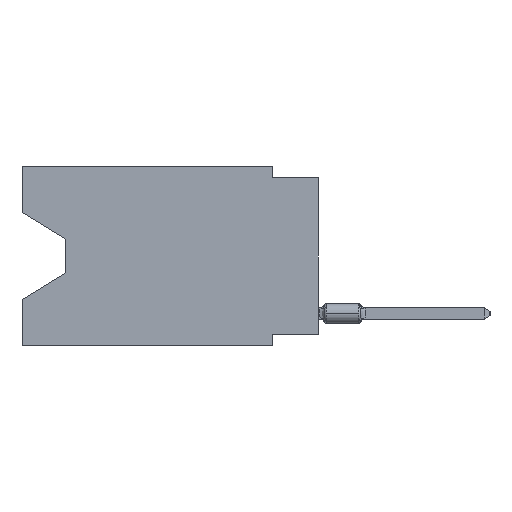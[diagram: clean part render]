
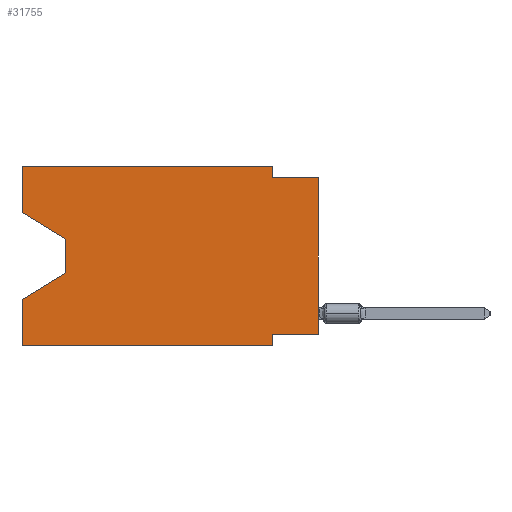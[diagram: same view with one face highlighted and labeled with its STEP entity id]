
A CAD part, left-side view. The second image highlights one B-rep face of the part: STEP entity #31755.
In plain terms, the highlighted planar face has unit normal (-1, 0, 0).
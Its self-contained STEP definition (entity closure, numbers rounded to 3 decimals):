
#3 = CARTESIAN_POINT ( 'NONE',  ( 0., 16.383, -2.546 ) ) ;
#266 = DIRECTION ( 'NONE',  ( 0., 0.855, -0.519 ) ) ;
#741 = EDGE_CURVE ( 'NONE', #55775, #19733, #58046, .T. ) ;
#993 = EDGE_CURVE ( 'NONE', #16217, #6384, #21470, .T. ) ;
#4747 = VECTOR ( 'NONE', #56675, 1000. ) ;
#5425 = EDGE_CURVE ( 'NONE', #16217, #34141, #39966, .T. ) ;
#5460 = EDGE_CURVE ( 'NONE', #55775, #35177, #15376, .T. ) ;
#5463 = CARTESIAN_POINT ( 'NONE',  ( 0., 2.54, 0. ) ) ;
#5688 = EDGE_CURVE ( 'NONE', #6384, #24599, #43544, .T. ) ;
#6215 = CARTESIAN_POINT ( 'NONE',  ( 0., 0., 0. ) ) ;
#6384 = VERTEX_POINT ( 'NONE', #26692 ) ;
#6504 = ORIENTED_EDGE ( 'NONE', *, *, #25379, .F. ) ;
#6637 = VERTEX_POINT ( 'NONE', #59790 ) ;
#7893 = DIRECTION ( 'NONE',  ( 0., 0., 1. ) ) ;
#8141 = LINE ( 'NONE', #43178, #21584 ) ;
#9099 = DIRECTION ( 'NONE',  ( 0., 0., -1. ) ) ;
#9825 = FACE_OUTER_BOUND ( 'NONE', #24979, .T. ) ;
#10461 = PLANE ( 'NONE',  #39262 ) ;
#12019 = CARTESIAN_POINT ( 'NONE',  ( 0., 16.383, -7.36 ) ) ;
#13508 = DIRECTION ( 'NONE',  ( 1., 0., 0. ) ) ;
#14356 = CARTESIAN_POINT ( 'NONE',  ( 0., 16.383, 0. ) ) ;
#14733 = VERTEX_POINT ( 'NONE', #24044 ) ;
#15062 = DIRECTION ( 'NONE',  ( 0., -0.855, -0.519 ) ) ;
#15376 = LINE ( 'NONE', #6215, #58860 ) ;
#15592 = LINE ( 'NONE', #5463, #54317 ) ;
#16217 = VERTEX_POINT ( 'NONE', #50211 ) ;
#17192 = CARTESIAN_POINT ( 'NONE',  ( 0., 16.383, 0. ) ) ;
#17951 = CARTESIAN_POINT ( 'NONE',  ( 0., 2.54, 0. ) ) ;
#18900 = DIRECTION ( 'NONE',  ( 0., -1., 0. ) ) ;
#19038 = VECTOR ( 'NONE', #53712, 1000. ) ;
#19636 = VERTEX_POINT ( 'NONE', #12019 ) ;
#19733 = VERTEX_POINT ( 'NONE', #49685 ) ;
#20646 = EDGE_CURVE ( 'NONE', #19733, #6637, #49858, .T. ) ;
#21047 = DIRECTION ( 'NONE',  ( 0., -1., 0. ) ) ;
#21470 = LINE ( 'NONE', #17192, #53207 ) ;
#21584 = VECTOR ( 'NONE', #18900, 1000. ) ;
#22934 = LINE ( 'NONE', #58698, #28875 ) ;
#23372 = ORIENTED_EDGE ( 'NONE', *, *, #61097, .T. ) ;
#23445 = ORIENTED_EDGE ( 'NONE', *, *, #51139, .T. ) ;
#23600 = EDGE_CURVE ( 'NONE', #24599, #28301, #15592, .T. ) ;
#23714 = ORIENTED_EDGE ( 'NONE', *, *, #49152, .F. ) ;
#24044 = CARTESIAN_POINT ( 'NONE',  ( 0., 13.97, -5.893 ) ) ;
#24599 = VERTEX_POINT ( 'NONE', #17951 ) ;
#24910 = CARTESIAN_POINT ( 'NONE',  ( 0., 2.54, -9.906 ) ) ;
#24979 = EDGE_LOOP ( 'NONE', ( #38047, #23445, #23372, #23714, #28029, #46603, #27506, #29976, #6504, #38285, #33761, #47927 ) ) ;
#25207 = CARTESIAN_POINT ( 'NONE',  ( 0., 0., -0.635 ) ) ;
#25379 = EDGE_CURVE ( 'NONE', #28301, #35177, #42009, .T. ) ;
#25544 = DIRECTION ( 'NONE',  ( 0., 0., 1. ) ) ;
#26692 = CARTESIAN_POINT ( 'NONE',  ( 0., 16.383, 0. ) ) ;
#27506 = ORIENTED_EDGE ( 'NONE', *, *, #741, .F. ) ;
#28029 = ORIENTED_EDGE ( 'NONE', *, *, #52487, .T. ) ;
#28301 = VERTEX_POINT ( 'NONE', #39928 ) ;
#28875 = VECTOR ( 'NONE', #7893, 1000. ) ;
#29799 = CARTESIAN_POINT ( 'NONE',  ( 0., 16.383, 0. ) ) ;
#29976 = ORIENTED_EDGE ( 'NONE', *, *, #5460, .T. ) ;
#31755 = ADVANCED_FACE ( 'NONE', ( #9825 ), #10461, .F. ) ;
#33484 = DIRECTION ( 'NONE',  ( 0., 0., -1. ) ) ;
#33761 = ORIENTED_EDGE ( 'NONE', *, *, #5688, .F. ) ;
#34141 = VERTEX_POINT ( 'NONE', #64300 ) ;
#34325 = VECTOR ( 'NONE', #43249, 1000. ) ;
#35177 = VERTEX_POINT ( 'NONE', #25207 ) ;
#35387 = CARTESIAN_POINT ( 'NONE',  ( 0., 0., -9.271 ) ) ;
#37346 = CARTESIAN_POINT ( 'NONE',  ( 0., 0., -9.271 ) ) ;
#38047 = ORIENTED_EDGE ( 'NONE', *, *, #5425, .T. ) ;
#38285 = ORIENTED_EDGE ( 'NONE', *, *, #23600, .F. ) ;
#39262 = AXIS2_PLACEMENT_3D ( 'NONE', #29799, #13508, #33484 ) ;
#39928 = CARTESIAN_POINT ( 'NONE',  ( 0., 2.54, -0.635 ) ) ;
#39966 = LINE ( 'NONE', #3, #53649 ) ;
#41779 = CARTESIAN_POINT ( 'NONE',  ( 0., 16.383, -9.906 ) ) ;
#41786 = DIRECTION ( 'NONE',  ( 0., 0., 1. ) ) ;
#42009 = LINE ( 'NONE', #61105, #47117 ) ;
#42565 = VECTOR ( 'NONE', #45898, 1000. ) ;
#43178 = CARTESIAN_POINT ( 'NONE',  ( 0., 16.383, -9.906 ) ) ;
#43249 = DIRECTION ( 'NONE',  ( 0., 1., 0. ) ) ;
#43544 = LINE ( 'NONE', #14356, #19038 ) ;
#44311 = VECTOR ( 'NONE', #266, 1000. ) ;
#45164 = CARTESIAN_POINT ( 'NONE',  ( 0., 13.97, -5.893 ) ) ;
#45898 = DIRECTION ( 'NONE',  ( 0., 0., -1. ) ) ;
#46603 = ORIENTED_EDGE ( 'NONE', *, *, #20646, .F. ) ;
#47117 = VECTOR ( 'NONE', #21047, 1000. ) ;
#47927 = ORIENTED_EDGE ( 'NONE', *, *, #993, .F. ) ;
#49147 = LINE ( 'NONE', #45164, #44311 ) ;
#49152 = EDGE_CURVE ( 'NONE', #58137, #19636, #22934, .T. ) ;
#49685 = CARTESIAN_POINT ( 'NONE',  ( 0., 2.54, -9.271 ) ) ;
#49858 = LINE ( 'NONE', #24910, #42565 ) ;
#50211 = CARTESIAN_POINT ( 'NONE',  ( 0., 16.383, -2.546 ) ) ;
#51139 = EDGE_CURVE ( 'NONE', #34141, #14733, #52055, .T. ) ;
#52055 = LINE ( 'NONE', #52376, #4747 ) ;
#52376 = CARTESIAN_POINT ( 'NONE',  ( 0., 13.97, -4.013 ) ) ;
#52487 = EDGE_CURVE ( 'NONE', #58137, #6637, #8141, .T. ) ;
#53207 = VECTOR ( 'NONE', #41786, 1000. ) ;
#53649 = VECTOR ( 'NONE', #15062, 1000. ) ;
#53712 = DIRECTION ( 'NONE',  ( 0., -1., 0. ) ) ;
#54317 = VECTOR ( 'NONE', #9099, 1000. ) ;
#55775 = VERTEX_POINT ( 'NONE', #35387 ) ;
#56675 = DIRECTION ( 'NONE',  ( 0., 0., -1. ) ) ;
#58046 = LINE ( 'NONE', #37346, #34325 ) ;
#58137 = VERTEX_POINT ( 'NONE', #41779 ) ;
#58698 = CARTESIAN_POINT ( 'NONE',  ( 0., 16.383, 0. ) ) ;
#58860 = VECTOR ( 'NONE', #25544, 1000. ) ;
#59790 = CARTESIAN_POINT ( 'NONE',  ( 0., 2.54, -9.906 ) ) ;
#61097 = EDGE_CURVE ( 'NONE', #14733, #19636, #49147, .T. ) ;
#61105 = CARTESIAN_POINT ( 'NONE',  ( 0., 0., -0.635 ) ) ;
#64300 = CARTESIAN_POINT ( 'NONE',  ( 0., 13.97, -4.013 ) ) ;
